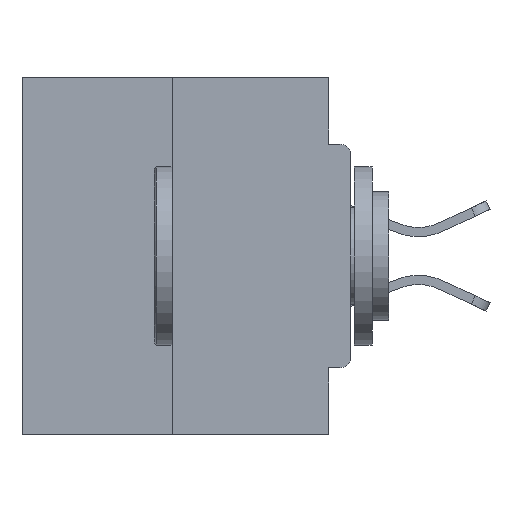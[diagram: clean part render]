
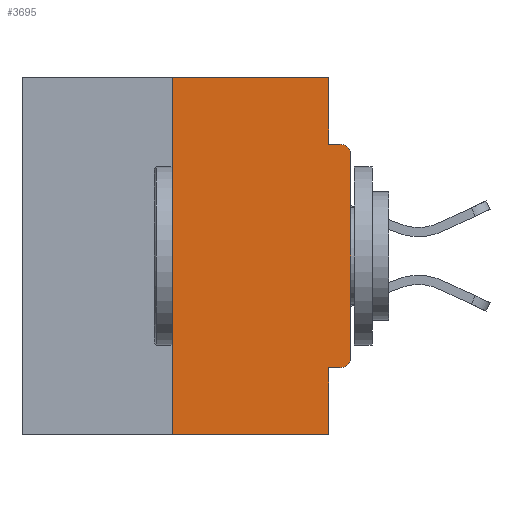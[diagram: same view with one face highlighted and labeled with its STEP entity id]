
A CAD part, left-side view. The second image highlights one B-rep face of the part: STEP entity #3695.
In plain terms, the highlighted planar face has unit normal (-1, 0, 0).
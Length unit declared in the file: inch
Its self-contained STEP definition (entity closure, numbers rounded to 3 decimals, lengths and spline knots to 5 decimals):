
#85 = EDGE_CURVE ( 'NONE', #9599, #24076, #7044, .T. ) ;
#214 = VECTOR ( 'NONE', #11160, 39.37008 ) ;
#330 = VERTEX_POINT ( 'NONE', #18555 ) ;
#464 = VECTOR ( 'NONE', #14755, 39.37008 ) ;
#658 = CARTESIAN_POINT ( 'NONE',  ( 0., 0.031, -0.5 ) ) ;
#884 = DIRECTION ( 'NONE',  ( 0., 1., 0. ) ) ;
#959 = LINE ( 'NONE', #34030, #17898 ) ;
#1309 = CARTESIAN_POINT ( 'NONE',  ( 0., 0.031, -0.4065 ) ) ;
#1338 = DIRECTION ( 'NONE',  ( 0., 0., -1. ) ) ;
#2046 = DIRECTION ( 'NONE',  ( -1., 0., 0. ) ) ;
#2119 = EDGE_CURVE ( 'NONE', #23917, #27002, #25488, .T. ) ;
#2504 = DIRECTION ( 'NONE',  ( 0., 0., -1. ) ) ;
#2989 = PLANE ( 'NONE',  #10844 ) ;
#3695 = ADVANCED_FACE ( 'NONE', ( #23719 ), #2989, .F. ) ;
#3742 = CARTESIAN_POINT ( 'NONE',  ( 0., 0.015, -0.0935 ) ) ;
#4122 = CARTESIAN_POINT ( 'NONE',  ( 0., 0., -0.1085 ) ) ;
#4437 = VECTOR ( 'NONE', #25483, 39.37008 ) ;
#4614 = DIRECTION ( 'NONE',  ( 1., 0., 0. ) ) ;
#5288 = LINE ( 'NONE', #28303, #10652 ) ;
#5527 = EDGE_CURVE ( 'NONE', #330, #23917, #8663, .T. ) ;
#6033 = LINE ( 'NONE', #21785, #30411 ) ;
#7023 = CARTESIAN_POINT ( 'NONE',  ( 0., 0., 0. ) ) ;
#7044 = LINE ( 'NONE', #19911, #464 ) ;
#7217 = LINE ( 'NONE', #10931, #214 ) ;
#8517 = VERTEX_POINT ( 'NONE', #14037 ) ;
#8559 = ORIENTED_EDGE ( 'NONE', *, *, #29048, .F. ) ;
#8663 = CIRCLE ( 'NONE', #22335, 0.015 ) ;
#9499 = DIRECTION ( 'NONE',  ( 0., 0., -1. ) ) ;
#9599 = VERTEX_POINT ( 'NONE', #10098 ) ;
#10098 = CARTESIAN_POINT ( 'NONE',  ( 0., 0.031, 0. ) ) ;
#10652 = VECTOR ( 'NONE', #20206, 39.37008 ) ;
#10826 = CARTESIAN_POINT ( 'NONE',  ( 0., 0.46, 0. ) ) ;
#10844 = AXIS2_PLACEMENT_3D ( 'NONE', #10826, #4614, #1338 ) ;
#10931 = CARTESIAN_POINT ( 'NONE',  ( 0., 0.46, -0.5 ) ) ;
#11160 = DIRECTION ( 'NONE',  ( 0., -1., 0. ) ) ;
#11903 = LINE ( 'NONE', #12251, #25090 ) ;
#12251 = CARTESIAN_POINT ( 'NONE',  ( 0., 0.031, -0.5 ) ) ;
#12281 = CARTESIAN_POINT ( 'NONE',  ( 0., 0., -0.3915 ) ) ;
#12404 = VERTEX_POINT ( 'NONE', #658 ) ;
#12466 = EDGE_CURVE ( 'NONE', #330, #21118, #6033, .T. ) ;
#12576 = CARTESIAN_POINT ( 'NONE',  ( 0., 0.015, -0.1085 ) ) ;
#12894 = LINE ( 'NONE', #23562, #26570 ) ;
#13200 = CARTESIAN_POINT ( 'NONE',  ( 0., 0.25, -0.5 ) ) ;
#14037 = CARTESIAN_POINT ( 'NONE',  ( 0., 0.25, 0. ) ) ;
#14103 = VERTEX_POINT ( 'NONE', #3742 ) ;
#14199 = ORIENTED_EDGE ( 'NONE', *, *, #31504, .T. ) ;
#14479 = EDGE_CURVE ( 'NONE', #24076, #14103, #12894, .T. ) ;
#14755 = DIRECTION ( 'NONE',  ( 0., 0., -1. ) ) ;
#14884 = ORIENTED_EDGE ( 'NONE', *, *, #85, .F. ) ;
#17892 = DIRECTION ( 'NONE',  ( 0., 0., -1. ) ) ;
#17898 = VECTOR ( 'NONE', #18181, 39.37008 ) ;
#18106 = ORIENTED_EDGE ( 'NONE', *, *, #25434, .F. ) ;
#18181 = DIRECTION ( 'NONE',  ( 0., 0., 1. ) ) ;
#18555 = CARTESIAN_POINT ( 'NONE',  ( 0., 0.015, -0.4065 ) ) ;
#19054 = ORIENTED_EDGE ( 'NONE', *, *, #25464, .F. ) ;
#19194 = ORIENTED_EDGE ( 'NONE', *, *, #20372, .T. ) ;
#19911 = CARTESIAN_POINT ( 'NONE',  ( 0., 0.031, 0. ) ) ;
#20206 = DIRECTION ( 'NONE',  ( 0., -1., 0. ) ) ;
#20352 = CIRCLE ( 'NONE', #20969, 0.015 ) ;
#20372 = EDGE_CURVE ( 'NONE', #27763, #12404, #7217, .T. ) ;
#20423 = DIRECTION ( 'NONE',  ( -1., 0., 0. ) ) ;
#20969 = AXIS2_PLACEMENT_3D ( 'NONE', #12576, #20423, #17892 ) ;
#21118 = VERTEX_POINT ( 'NONE', #1309 ) ;
#21785 = CARTESIAN_POINT ( 'NONE',  ( 0., 0., -0.4065 ) ) ;
#22335 = AXIS2_PLACEMENT_3D ( 'NONE', #28607, #2046, #2504 ) ;
#23127 = ORIENTED_EDGE ( 'NONE', *, *, #12466, .F. ) ;
#23456 = ORIENTED_EDGE ( 'NONE', *, *, #14479, .F. ) ;
#23562 = CARTESIAN_POINT ( 'NONE',  ( 0., 0., -0.0935 ) ) ;
#23620 = EDGE_LOOP ( 'NONE', ( #18106, #8559, #19194, #19054, #23127, #31124, #29974, #14199, #23456, #14884 ) ) ;
#23719 = FACE_OUTER_BOUND ( 'NONE', #23620, .T. ) ;
#23917 = VERTEX_POINT ( 'NONE', #12281 ) ;
#24076 = VERTEX_POINT ( 'NONE', #28673 ) ;
#25090 = VECTOR ( 'NONE', #9499, 39.37008 ) ;
#25434 = EDGE_CURVE ( 'NONE', #8517, #9599, #5288, .T. ) ;
#25464 = EDGE_CURVE ( 'NONE', #21118, #12404, #11903, .T. ) ;
#25483 = DIRECTION ( 'NONE',  ( 0., 0., 1. ) ) ;
#25488 = LINE ( 'NONE', #7023, #4437 ) ;
#26570 = VECTOR ( 'NONE', #34141, 39.37008 ) ;
#27002 = VERTEX_POINT ( 'NONE', #4122 ) ;
#27763 = VERTEX_POINT ( 'NONE', #13200 ) ;
#28303 = CARTESIAN_POINT ( 'NONE',  ( 0., 0.46, 0. ) ) ;
#28607 = CARTESIAN_POINT ( 'NONE',  ( 0., 0.015, -0.3915 ) ) ;
#28673 = CARTESIAN_POINT ( 'NONE',  ( 0., 0.031, -0.0935 ) ) ;
#29048 = EDGE_CURVE ( 'NONE', #27763, #8517, #959, .T. ) ;
#29974 = ORIENTED_EDGE ( 'NONE', *, *, #2119, .T. ) ;
#30411 = VECTOR ( 'NONE', #884, 39.37008 ) ;
#31124 = ORIENTED_EDGE ( 'NONE', *, *, #5527, .T. ) ;
#31504 = EDGE_CURVE ( 'NONE', #27002, #14103, #20352, .T. ) ;
#34030 = CARTESIAN_POINT ( 'NONE',  ( 0., 0.25, 0. ) ) ;
#34141 = DIRECTION ( 'NONE',  ( 0., -1., 0. ) ) ;
